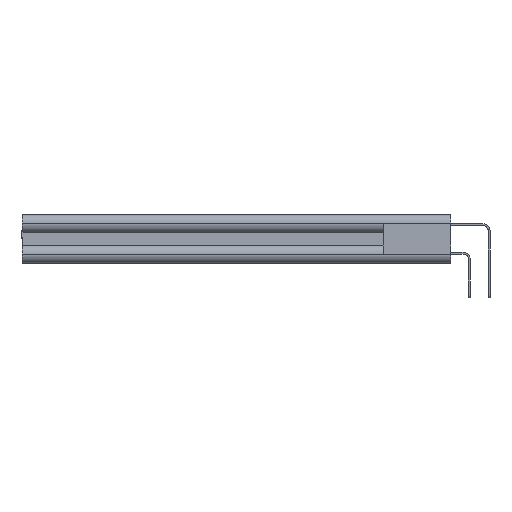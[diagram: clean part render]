
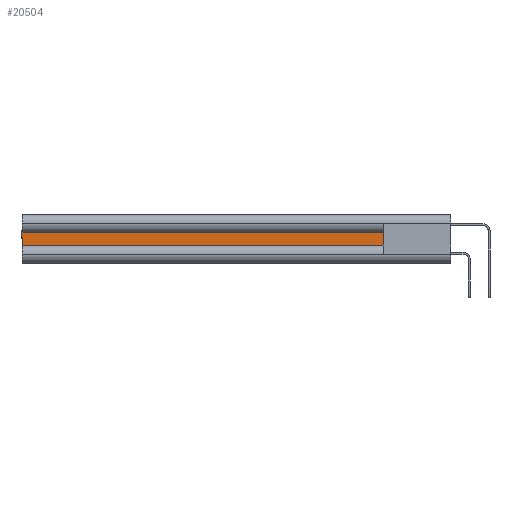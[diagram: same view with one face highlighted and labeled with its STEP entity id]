
A CAD part, left-side view. The second image highlights one B-rep face of the part: STEP entity #20504.
In plain terms, the highlighted planar face has unit normal (-1, 0, 0).
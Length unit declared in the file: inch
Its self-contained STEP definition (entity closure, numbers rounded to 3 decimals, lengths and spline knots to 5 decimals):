
#13 = DIRECTION ( 'NONE',  ( 0., 0., -1. ) ) ;
#194 = VERTEX_POINT ( 'NONE', #18633 ) ;
#364 = VERTEX_POINT ( 'NONE', #14564 ) ;
#749 = CARTESIAN_POINT ( 'NONE',  ( 0.044, 0.37012, 0.0465 ) ) ;
#798 = ORIENTED_EDGE ( 'NONE', *, *, #21369, .T. ) ;
#1427 = FACE_OUTER_BOUND ( 'NONE', #3785, .T. ) ;
#2399 = VECTOR ( 'NONE', #20812, 39.37008 ) ;
#2754 = CARTESIAN_POINT ( 'NONE',  ( 0.044, 0.473, -0.0465 ) ) ;
#3546 = VECTOR ( 'NONE', #17166, 39.37008 ) ;
#3574 = DIRECTION ( 'NONE',  ( 0., 1., 0. ) ) ;
#3785 = EDGE_LOOP ( 'NONE', ( #798, #17836, #12257, #15298 ) ) ;
#4617 = VERTEX_POINT ( 'NONE', #13938 ) ;
#6244 = VECTOR ( 'NONE', #22313, 39.37008 ) ;
#6615 = VERTEX_POINT ( 'NONE', #20001 ) ;
#7508 = EDGE_CURVE ( 'NONE', #6615, #364, #13122, .T. ) ;
#7802 = LINE ( 'NONE', #13711, #2399 ) ;
#8957 = CARTESIAN_POINT ( 'NONE',  ( 0.044, 0.37012, -0.0465 ) ) ;
#9131 = PLANE ( 'NONE',  #10332 ) ;
#10332 = AXIS2_PLACEMENT_3D ( 'NONE', #19829, #10924, #13 ) ;
#10440 = VECTOR ( 'NONE', #3574, 39.37008 ) ;
#10924 = DIRECTION ( 'NONE',  ( 1., 0., 0. ) ) ;
#11557 = LINE ( 'NONE', #8957, #10440 ) ;
#12257 = ORIENTED_EDGE ( 'NONE', *, *, #13935, .F. ) ;
#13122 = LINE ( 'NONE', #2754, #3546 ) ;
#13711 = CARTESIAN_POINT ( 'NONE',  ( 0.044, 3., -0.0465 ) ) ;
#13935 = EDGE_CURVE ( 'NONE', #364, #194, #11557, .T. ) ;
#13938 = CARTESIAN_POINT ( 'NONE',  ( 0.044, 3., 0.0465 ) ) ;
#14564 = CARTESIAN_POINT ( 'NONE',  ( 0.044, 0.473, -0.0465 ) ) ;
#15298 = ORIENTED_EDGE ( 'NONE', *, *, #7508, .F. ) ;
#15848 = EDGE_CURVE ( 'NONE', #4617, #194, #7802, .T. ) ;
#17166 = DIRECTION ( 'NONE',  ( 0., 0., -1. ) ) ;
#17836 = ORIENTED_EDGE ( 'NONE', *, *, #15848, .T. ) ;
#18633 = CARTESIAN_POINT ( 'NONE',  ( 0.044, 3., -0.0465 ) ) ;
#19829 = CARTESIAN_POINT ( 'NONE',  ( 0.044, 0.37012, -0.0465 ) ) ;
#20001 = CARTESIAN_POINT ( 'NONE',  ( 0.044, 0.473, 0.0465 ) ) ;
#20504 = ADVANCED_FACE ( 'NONE', ( #1427 ), #9131, .F. ) ;
#20527 = LINE ( 'NONE', #749, #6244 ) ;
#20812 = DIRECTION ( 'NONE',  ( 0., 0., -1. ) ) ;
#21369 = EDGE_CURVE ( 'NONE', #6615, #4617, #20527, .T. ) ;
#22313 = DIRECTION ( 'NONE',  ( 0., 1., 0. ) ) ;
